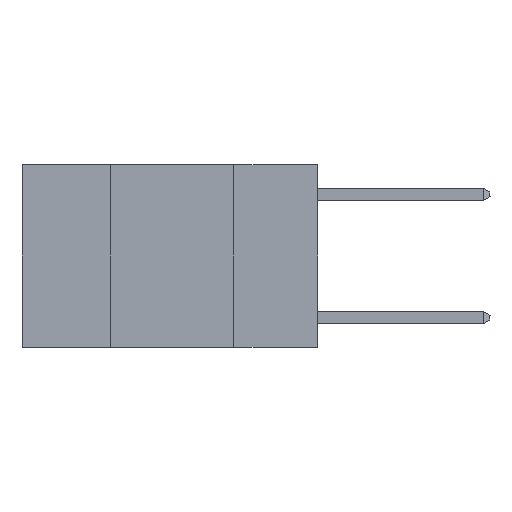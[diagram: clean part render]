
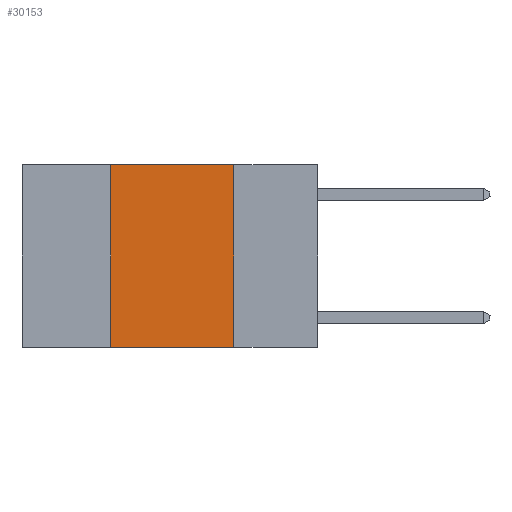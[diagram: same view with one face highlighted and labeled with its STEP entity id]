
A CAD part, left-side view. The second image highlights one B-rep face of the part: STEP entity #30153.
In plain terms, the highlighted planar face has unit normal (-1, 0, 0).
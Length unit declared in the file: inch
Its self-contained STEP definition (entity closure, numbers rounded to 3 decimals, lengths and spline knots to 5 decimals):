
#1483 = VECTOR ( 'NONE', #20643, 39.37008 ) ;
#1919 = VECTOR ( 'NONE', #10346, 39.37008 ) ;
#2761 = CARTESIAN_POINT ( 'NONE',  ( 0., 0.6, 0. ) ) ;
#2991 = VECTOR ( 'NONE', #10950, 39.37008 ) ;
#4268 = DIRECTION ( 'NONE',  ( 1., 0., 0. ) ) ;
#4825 = ORIENTED_EDGE ( 'NONE', *, *, #23164, .T. ) ;
#6565 = ORIENTED_EDGE ( 'NONE', *, *, #10451, .F. ) ;
#8172 = CARTESIAN_POINT ( 'NONE',  ( 0., 0.17, 0. ) ) ;
#8197 = VERTEX_POINT ( 'NONE', #13488 ) ;
#8961 = CARTESIAN_POINT ( 'NONE',  ( 0., 0.17, 0. ) ) ;
#9894 = EDGE_CURVE ( 'NONE', #12440, #8197, #20479, .T. ) ;
#10346 = DIRECTION ( 'NONE',  ( 0., -1., 0. ) ) ;
#10451 = EDGE_CURVE ( 'NONE', #30453, #13566, #18965, .T. ) ;
#10950 = DIRECTION ( 'NONE',  ( 0., 0., -1. ) ) ;
#11349 = ORIENTED_EDGE ( 'NONE', *, *, #25308, .F. ) ;
#12440 = VERTEX_POINT ( 'NONE', #19515 ) ;
#13177 = CARTESIAN_POINT ( 'NONE',  ( 0., 0.17, -0.37 ) ) ;
#13488 = CARTESIAN_POINT ( 'NONE',  ( 0., 0.42, 0. ) ) ;
#13566 = VERTEX_POINT ( 'NONE', #13177 ) ;
#15589 = CARTESIAN_POINT ( 'NONE',  ( 0., 0.42, 0. ) ) ;
#16705 = ORIENTED_EDGE ( 'NONE', *, *, #9894, .F. ) ;
#16776 = CARTESIAN_POINT ( 'NONE',  ( 0., 0.6, 0. ) ) ;
#18965 = LINE ( 'NONE', #8961, #2991 ) ;
#19366 = EDGE_LOOP ( 'NONE', ( #6565, #11349, #16705, #4825 ) ) ;
#19515 = CARTESIAN_POINT ( 'NONE',  ( 0., 0.42, -0.37 ) ) ;
#20479 = LINE ( 'NONE', #15589, #1483 ) ;
#20643 = DIRECTION ( 'NONE',  ( 0., 0., 1. ) ) ;
#21812 = FACE_OUTER_BOUND ( 'NONE', #19366, .T. ) ;
#23164 = EDGE_CURVE ( 'NONE', #12440, #13566, #24637, .T. ) ;
#24637 = LINE ( 'NONE', #27124, #29069 ) ;
#25092 = AXIS2_PLACEMENT_3D ( 'NONE', #16776, #4268, #31492 ) ;
#25308 = EDGE_CURVE ( 'NONE', #8197, #30453, #27861, .T. ) ;
#26402 = PLANE ( 'NONE',  #25092 ) ;
#27124 = CARTESIAN_POINT ( 'NONE',  ( 0., 0.6, -0.37 ) ) ;
#27861 = LINE ( 'NONE', #2761, #1919 ) ;
#29069 = VECTOR ( 'NONE', #30049, 39.37008 ) ;
#30049 = DIRECTION ( 'NONE',  ( 0., -1., 0. ) ) ;
#30153 = ADVANCED_FACE ( 'NONE', ( #21812 ), #26402, .F. ) ;
#30453 = VERTEX_POINT ( 'NONE', #8172 ) ;
#31492 = DIRECTION ( 'NONE',  ( 0., 0., -1. ) ) ;
